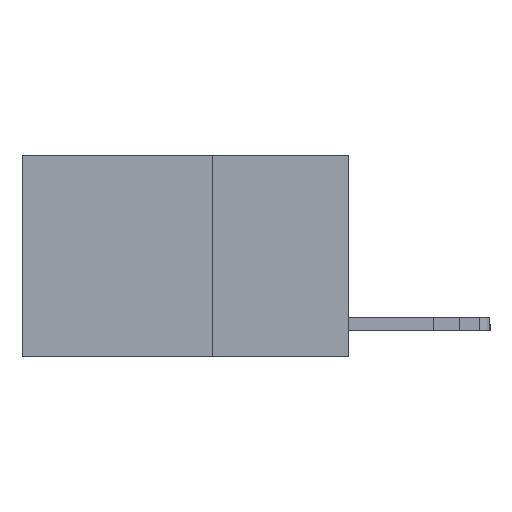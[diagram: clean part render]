
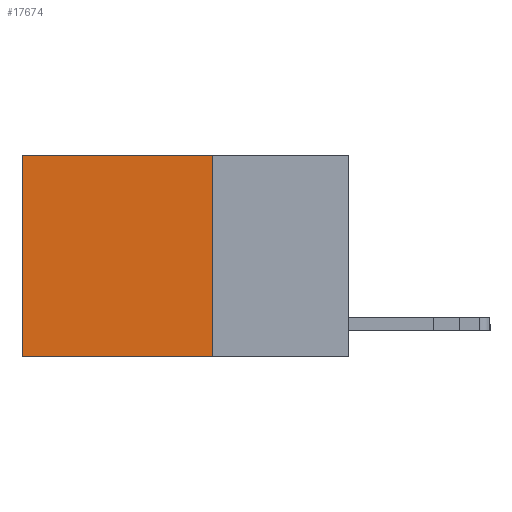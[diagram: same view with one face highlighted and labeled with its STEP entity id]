
A CAD part, left-side view. The second image highlights one B-rep face of the part: STEP entity #17674.
In plain terms, the highlighted planar face has unit normal (-1, 0, 0).
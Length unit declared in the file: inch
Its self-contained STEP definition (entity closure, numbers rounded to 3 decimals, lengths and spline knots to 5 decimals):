
#34 = DIRECTION ( 'NONE',  ( 0., 0., -1. ) ) ;
#286 = CARTESIAN_POINT ( 'NONE',  ( 0.2625, 0.25, 0. ) ) ;
#682 = VERTEX_POINT ( 'NONE', #1384 ) ;
#1144 = CARTESIAN_POINT ( 'NONE',  ( 0.2625, 0.25, -0.37 ) ) ;
#1384 = CARTESIAN_POINT ( 'NONE',  ( 0.2625, 0.25, 0. ) ) ;
#2908 = VECTOR ( 'NONE', #16741, 39.37008 ) ;
#3558 = CARTESIAN_POINT ( 'NONE',  ( 0.2625, 0.6, 0. ) ) ;
#4005 = AXIS2_PLACEMENT_3D ( 'NONE', #17741, #21142, #16157 ) ;
#4119 = VERTEX_POINT ( 'NONE', #20021 ) ;
#4334 = FACE_OUTER_BOUND ( 'NONE', #14699, .T. ) ;
#4816 = LINE ( 'NONE', #16970, #2908 ) ;
#5705 = ORIENTED_EDGE ( 'NONE', *, *, #17490, .T. ) ;
#7576 = LINE ( 'NONE', #16365, #14608 ) ;
#7794 = DIRECTION ( 'NONE',  ( 0., 1., 0. ) ) ;
#9803 = CARTESIAN_POINT ( 'NONE',  ( 0.2625, 0.6, 0. ) ) ;
#10370 = ORIENTED_EDGE ( 'NONE', *, *, #11088, .T. ) ;
#10378 = ORIENTED_EDGE ( 'NONE', *, *, #17154, .F. ) ;
#11088 = EDGE_CURVE ( 'NONE', #21836, #4119, #20603, .T. ) ;
#12606 = VERTEX_POINT ( 'NONE', #1144 ) ;
#14569 = PLANE ( 'NONE',  #4005 ) ;
#14608 = VECTOR ( 'NONE', #7794, 39.37008 ) ;
#14699 = EDGE_LOOP ( 'NONE', ( #10370, #21744, #10378, #5705 ) ) ;
#15854 = DIRECTION ( 'NONE',  ( 0., 0., -1. ) ) ;
#16157 = DIRECTION ( 'NONE',  ( 0., 0., -1. ) ) ;
#16365 = CARTESIAN_POINT ( 'NONE',  ( 0.2625, 0.25, -0.37 ) ) ;
#16436 = VECTOR ( 'NONE', #34, 39.37008 ) ;
#16741 = DIRECTION ( 'NONE',  ( 0., 1., 0. ) ) ;
#16970 = CARTESIAN_POINT ( 'NONE',  ( 0.2625, 0.25, 0. ) ) ;
#17154 = EDGE_CURVE ( 'NONE', #682, #12606, #20855, .T. ) ;
#17490 = EDGE_CURVE ( 'NONE', #682, #21836, #4816, .T. ) ;
#17674 = ADVANCED_FACE ( 'NONE', ( #4334 ), #14569, .F. ) ;
#17741 = CARTESIAN_POINT ( 'NONE',  ( 0.2625, 0.25, 0. ) ) ;
#19473 = VECTOR ( 'NONE', #15854, 39.37008 ) ;
#20010 = EDGE_CURVE ( 'NONE', #12606, #4119, #7576, .T. ) ;
#20021 = CARTESIAN_POINT ( 'NONE',  ( 0.2625, 0.6, -0.37 ) ) ;
#20603 = LINE ( 'NONE', #3558, #16436 ) ;
#20855 = LINE ( 'NONE', #286, #19473 ) ;
#21142 = DIRECTION ( 'NONE',  ( 1., 0., 0. ) ) ;
#21744 = ORIENTED_EDGE ( 'NONE', *, *, #20010, .F. ) ;
#21836 = VERTEX_POINT ( 'NONE', #9803 ) ;
